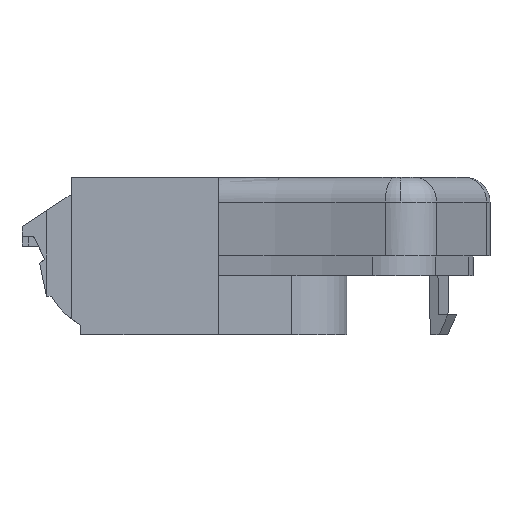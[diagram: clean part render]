
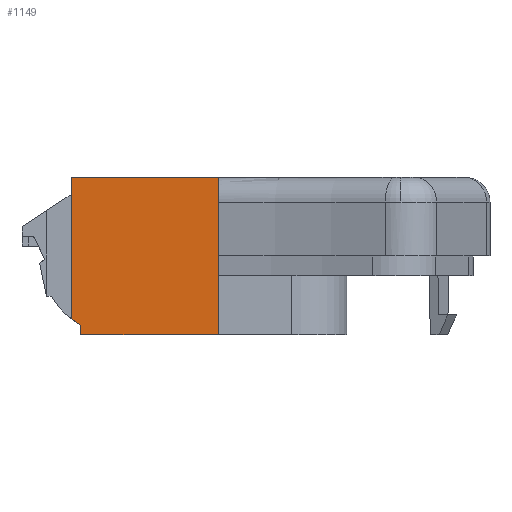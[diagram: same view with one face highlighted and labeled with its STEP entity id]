
A CAD part, left-side view. The second image highlights one B-rep face of the part: STEP entity #1149.
In plain terms, the highlighted planar face has unit normal (-0.999, 0.035, 0).
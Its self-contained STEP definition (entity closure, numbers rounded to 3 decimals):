
#36 = EDGE_CURVE ( 'NONE', #3631, #3008, #5702, .T. ) ;
#44 = VERTEX_POINT ( 'NONE', #1207 ) ;
#63 = CARTESIAN_POINT ( 'NONE',  ( -21.556, 2., 12.5 ) ) ;
#136 = CARTESIAN_POINT ( 'NONE',  ( -22.603, -28., 16. ) ) ;
#367 = LINE ( 'NONE', #3338, #3160 ) ;
#460 = FACE_OUTER_BOUND ( 'NONE', #3646, .T. ) ;
#504 = VERTEX_POINT ( 'NONE', #2443 ) ;
#597 = ORIENTED_EDGE ( 'NONE', *, *, #36, .T. ) ;
#798 = CARTESIAN_POINT ( 'NONE',  ( -21.508, 3.359, 16. ) ) ;
#821 = VERTEX_POINT ( 'NONE', #136 ) ;
#840 = CARTESIAN_POINT ( 'NONE',  ( -22.603, -28., -16. ) ) ;
#892 = DIRECTION ( 'NONE',  ( -0.035, -0.999, 0. ) ) ;
#913 = ORIENTED_EDGE ( 'NONE', *, *, #2061, .T. ) ;
#957 = DIRECTION ( 'NONE',  ( 0., 0., -1. ) ) ;
#1066 = LINE ( 'NONE', #1521, #3468 ) ;
#1149 = ADVANCED_FACE ( 'NONE', ( #460 ), #4886, .T. ) ;
#1207 = CARTESIAN_POINT ( 'NONE',  ( -21.625, 0., -16. ) ) ;
#1218 = LINE ( 'NONE', #1612, #4459 ) ;
#1263 = CARTESIAN_POINT ( 'NONE',  ( -21.578, 1.367, -13.288 ) ) ;
#1521 = CARTESIAN_POINT ( 'NONE',  ( -21.625, 0., -16. ) ) ;
#1595 = DIRECTION ( 'NONE',  ( -0.035, -0.999, 0. ) ) ;
#1612 = CARTESIAN_POINT ( 'NONE',  ( -22.603, -28., -16. ) ) ;
#1797 = LINE ( 'NONE', #798, #3874 ) ;
#2061 = EDGE_CURVE ( 'NONE', #821, #504, #1797, .T. ) ;
#2151 = CARTESIAN_POINT ( 'NONE',  ( -21.601, 0.699, -13.734 ) ) ;
#2333 = ORIENTED_EDGE ( 'NONE', *, *, #5482, .T. ) ;
#2442 = ORIENTED_EDGE ( 'NONE', *, *, #3517, .T. ) ;
#2443 = CARTESIAN_POINT ( 'NONE',  ( -21.556, 2., 16. ) ) ;
#2602 = VERTEX_POINT ( 'NONE', #4009 ) ;
#2846 = DIRECTION ( 'NONE',  ( 0., 0., -1. ) ) ;
#3008 = VERTEX_POINT ( 'NONE', #4810 ) ;
#3024 = LINE ( 'NONE', #63, #4986 ) ;
#3160 = VECTOR ( 'NONE', #1595, 1000. ) ;
#3287 = EDGE_CURVE ( 'NONE', #3008, #44, #1066, .T. ) ;
#3338 = CARTESIAN_POINT ( 'NONE',  ( -22.554, -26.605, -16. ) ) ;
#3459 = CARTESIAN_POINT ( 'NONE',  ( -21.556, 2., -12.793 ) ) ;
#3468 = VECTOR ( 'NONE', #2846, 1000. ) ;
#3517 = EDGE_CURVE ( 'NONE', #2602, #821, #1218, .T. ) ;
#3631 = VERTEX_POINT ( 'NONE', #3459 ) ;
#3646 = EDGE_LOOP ( 'NONE', ( #2333, #597, #4051, #3863, #2442, #913 ) ) ;
#3863 = ORIENTED_EDGE ( 'NONE', *, *, #5315, .T. ) ;
#3874 = VECTOR ( 'NONE', #4776, 1000. ) ;
#3898 = CARTESIAN_POINT ( 'NONE',  ( -21.556, 2., -12.793 ) ) ;
#4009 = CARTESIAN_POINT ( 'NONE',  ( -22.603, -28., -16. ) ) ;
#4051 = ORIENTED_EDGE ( 'NONE', *, *, #3287, .T. ) ;
#4349 = CARTESIAN_POINT ( 'NONE',  ( -21.625, 0., -14.13 ) ) ;
#4408 = AXIS2_PLACEMENT_3D ( 'NONE', #840, #5287, #892 ) ;
#4459 = VECTOR ( 'NONE', #4746, 1000. ) ;
#4746 = DIRECTION ( 'NONE',  ( 0., 0., 1. ) ) ;
#4776 = DIRECTION ( 'NONE',  ( 0.035, 0.999, 0. ) ) ;
#4810 = CARTESIAN_POINT ( 'NONE',  ( -21.625, 0., -14.13 ) ) ;
#4886 = PLANE ( 'NONE',  #4408 ) ;
#4986 = VECTOR ( 'NONE', #957, 1000. ) ;
#5287 = DIRECTION ( 'NONE',  ( -0.999, 0.035, 0. ) ) ;
#5315 = EDGE_CURVE ( 'NONE', #44, #2602, #367, .T. ) ;
#5482 = EDGE_CURVE ( 'NONE', #504, #3631, #3024, .T. ) ;
#5702 =( BOUNDED_CURVE ( )  B_SPLINE_CURVE ( 3, ( #3898, #1263, #2151, #4349 ),
 .UNSPECIFIED., .F., .F. ) 
 B_SPLINE_CURVE_WITH_KNOTS ( ( 4, 4 ),
 ( 4.049, 4.197 ),
 .UNSPECIFIED. ) 
 CURVE ( )  GEOMETRIC_REPRESENTATION_ITEM ( )  RATIONAL_B_SPLINE_CURVE ( ( 1., 0.998, 0.998, 1. ) ) 
 REPRESENTATION_ITEM ( '' )  );
